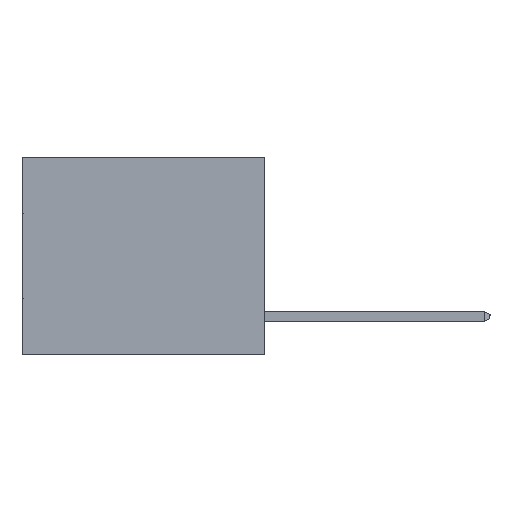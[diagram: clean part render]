
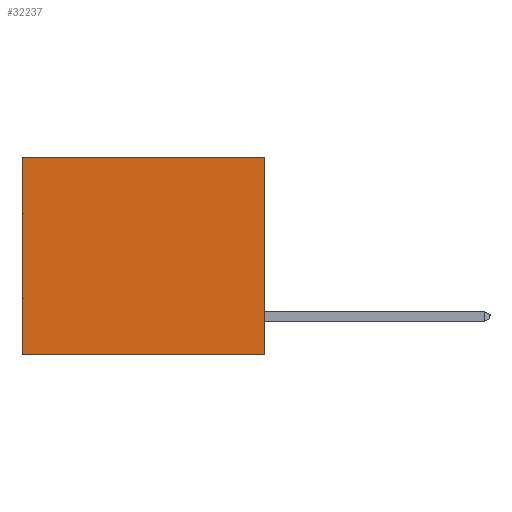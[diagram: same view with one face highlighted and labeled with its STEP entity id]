
A CAD part, left-side view. The second image highlights one B-rep face of the part: STEP entity #32237.
In plain terms, the highlighted planar face has unit normal (-1, 0, 0).
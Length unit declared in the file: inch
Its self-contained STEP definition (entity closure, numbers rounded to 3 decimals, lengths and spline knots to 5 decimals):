
#93 = CARTESIAN_POINT ( 'NONE',  ( 0.3165, 0.6, -0.49 ) ) ;
#1640 = FACE_OUTER_BOUND ( 'NONE', #14976, .T. ) ;
#2707 = VERTEX_POINT ( 'NONE', #93 ) ;
#5341 = VECTOR ( 'NONE', #7964, 39.37008 ) ;
#5688 = EDGE_CURVE ( 'NONE', #29249, #17513, #30027, .T. ) ;
#5812 = ORIENTED_EDGE ( 'NONE', *, *, #22647, .F. ) ;
#6686 = EDGE_CURVE ( 'NONE', #29249, #31106, #12446, .T. ) ;
#6764 = LINE ( 'NONE', #17136, #31372 ) ;
#6843 = AXIS2_PLACEMENT_3D ( 'NONE', #25779, #15202, #33825 ) ;
#7964 = DIRECTION ( 'NONE',  ( 0., 0., -1. ) ) ;
#12263 = CARTESIAN_POINT ( 'NONE',  ( 0.3165, 0.6, 0. ) ) ;
#12446 = LINE ( 'NONE', #15685, #5341 ) ;
#13233 = CARTESIAN_POINT ( 'NONE',  ( 0.3165, 0., -0.49 ) ) ;
#14792 = DIRECTION ( 'NONE',  ( 0., 0., -1. ) ) ;
#14976 = EDGE_LOOP ( 'NONE', ( #15820, #5812, #16617, #30592 ) ) ;
#15202 = DIRECTION ( 'NONE',  ( 1., 0., 0. ) ) ;
#15392 = CARTESIAN_POINT ( 'NONE',  ( 0.3165, 0., 0. ) ) ;
#15685 = CARTESIAN_POINT ( 'NONE',  ( 0.3165, 0., -0.49 ) ) ;
#15820 = ORIENTED_EDGE ( 'NONE', *, *, #22857, .T. ) ;
#16086 = CARTESIAN_POINT ( 'NONE',  ( 0.3165, 0., -0.49 ) ) ;
#16617 = ORIENTED_EDGE ( 'NONE', *, *, #6686, .F. ) ;
#16806 = LINE ( 'NONE', #16086, #28911 ) ;
#17136 = CARTESIAN_POINT ( 'NONE',  ( 0.3165, 0.6, -0.49 ) ) ;
#17478 = DIRECTION ( 'NONE',  ( 0., 1., 0. ) ) ;
#17513 = VERTEX_POINT ( 'NONE', #12263 ) ;
#22503 = CARTESIAN_POINT ( 'NONE',  ( 0.3165, 0., 0. ) ) ;
#22647 = EDGE_CURVE ( 'NONE', #31106, #2707, #16806, .T. ) ;
#22857 = EDGE_CURVE ( 'NONE', #17513, #2707, #6764, .T. ) ;
#25557 = PLANE ( 'NONE',  #6843 ) ;
#25779 = CARTESIAN_POINT ( 'NONE',  ( 0.3165, 0., -0.49 ) ) ;
#26562 = DIRECTION ( 'NONE',  ( 0., 1., 0. ) ) ;
#28833 = VECTOR ( 'NONE', #17478, 39.37008 ) ;
#28911 = VECTOR ( 'NONE', #26562, 39.37008 ) ;
#29249 = VERTEX_POINT ( 'NONE', #15392 ) ;
#30027 = LINE ( 'NONE', #22503, #28833 ) ;
#30592 = ORIENTED_EDGE ( 'NONE', *, *, #5688, .T. ) ;
#31106 = VERTEX_POINT ( 'NONE', #13233 ) ;
#31372 = VECTOR ( 'NONE', #14792, 39.37008 ) ;
#32237 = ADVANCED_FACE ( 'NONE', ( #1640 ), #25557, .F. ) ;
#33825 = DIRECTION ( 'NONE',  ( 0., 0., -1. ) ) ;
